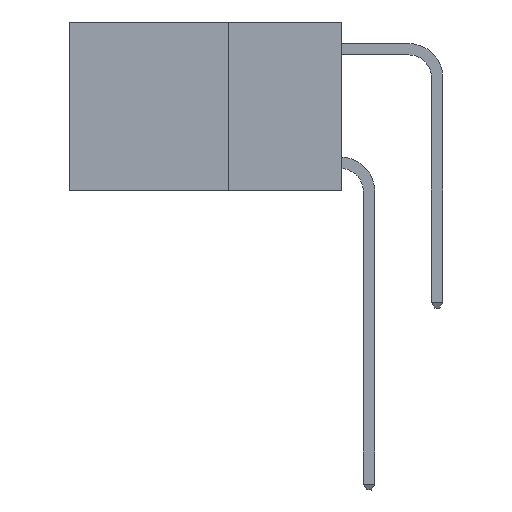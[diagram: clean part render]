
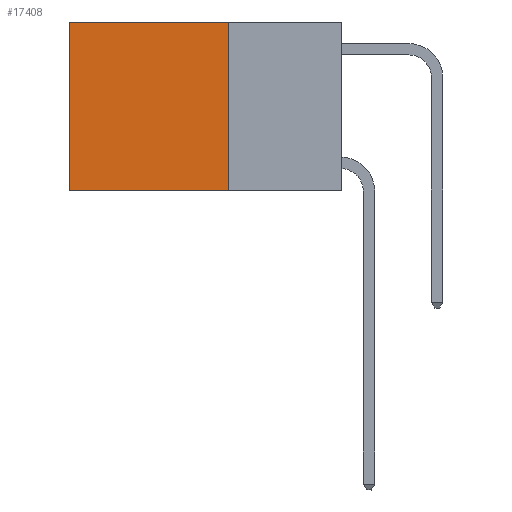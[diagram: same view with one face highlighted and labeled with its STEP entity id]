
A CAD part, left-side view. The second image highlights one B-rep face of the part: STEP entity #17408.
In plain terms, the highlighted planar face has unit normal (-1, 0, 0).
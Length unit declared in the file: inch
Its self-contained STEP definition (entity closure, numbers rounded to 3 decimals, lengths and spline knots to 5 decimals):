
#525 = CARTESIAN_POINT ( 'NONE',  ( 0.2625, 0.25, -0.37 ) ) ;
#909 = CARTESIAN_POINT ( 'NONE',  ( 0.2625, 0.25, -0.37 ) ) ;
#1007 = VECTOR ( 'NONE', #11869, 39.37008 ) ;
#1152 = DIRECTION ( 'NONE',  ( 0., 0., -1. ) ) ;
#2261 = VECTOR ( 'NONE', #1152, 39.37008 ) ;
#2511 = DIRECTION ( 'NONE',  ( 1., 0., 0. ) ) ;
#2777 = CARTESIAN_POINT ( 'NONE',  ( 0.2625, 0.6, 0. ) ) ;
#4177 = VERTEX_POINT ( 'NONE', #11065 ) ;
#4602 = FACE_OUTER_BOUND ( 'NONE', #7249, .T. ) ;
#4671 = ORIENTED_EDGE ( 'NONE', *, *, #17528, .F. ) ;
#5500 = CARTESIAN_POINT ( 'NONE',  ( 0.2625, 0.6, 0. ) ) ;
#6411 = ORIENTED_EDGE ( 'NONE', *, *, #17783, .T. ) ;
#6715 = PLANE ( 'NONE',  #9550 ) ;
#7249 = EDGE_LOOP ( 'NONE', ( #20019, #4671, #20841, #6411 ) ) ;
#9550 = AXIS2_PLACEMENT_3D ( 'NONE', #14649, #2511, #12687 ) ;
#10264 = VECTOR ( 'NONE', #19568, 39.37008 ) ;
#11065 = CARTESIAN_POINT ( 'NONE',  ( 0.2625, 0.6, -0.37 ) ) ;
#11152 = EDGE_CURVE ( 'NONE', #14531, #4177, #19249, .T. ) ;
#11294 = VERTEX_POINT ( 'NONE', #22407 ) ;
#11869 = DIRECTION ( 'NONE',  ( 0., 1., 0. ) ) ;
#12687 = DIRECTION ( 'NONE',  ( 0., 0., -1. ) ) ;
#13375 = LINE ( 'NONE', #19695, #10264 ) ;
#13833 = LINE ( 'NONE', #23856, #1007 ) ;
#14226 = EDGE_CURVE ( 'NONE', #11294, #17500, #13375, .T. ) ;
#14531 = VERTEX_POINT ( 'NONE', #2777 ) ;
#14649 = CARTESIAN_POINT ( 'NONE',  ( 0.2625, 0.25, 0. ) ) ;
#17141 = VECTOR ( 'NONE', #25046, 39.37008 ) ;
#17408 = ADVANCED_FACE ( 'NONE', ( #4602 ), #6715, .F. ) ;
#17500 = VERTEX_POINT ( 'NONE', #525 ) ;
#17528 = EDGE_CURVE ( 'NONE', #17500, #4177, #24790, .T. ) ;
#17783 = EDGE_CURVE ( 'NONE', #11294, #14531, #13833, .T. ) ;
#19249 = LINE ( 'NONE', #5500, #2261 ) ;
#19568 = DIRECTION ( 'NONE',  ( 0., 0., -1. ) ) ;
#19695 = CARTESIAN_POINT ( 'NONE',  ( 0.2625, 0.25, 0. ) ) ;
#20019 = ORIENTED_EDGE ( 'NONE', *, *, #11152, .T. ) ;
#20841 = ORIENTED_EDGE ( 'NONE', *, *, #14226, .F. ) ;
#22407 = CARTESIAN_POINT ( 'NONE',  ( 0.2625, 0.25, 0. ) ) ;
#23856 = CARTESIAN_POINT ( 'NONE',  ( 0.2625, 0.25, 0. ) ) ;
#24790 = LINE ( 'NONE', #909, #17141 ) ;
#25046 = DIRECTION ( 'NONE',  ( 0., 1., 0. ) ) ;
